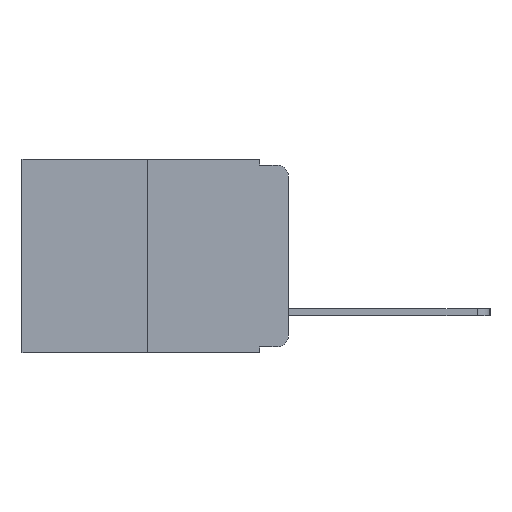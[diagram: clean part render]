
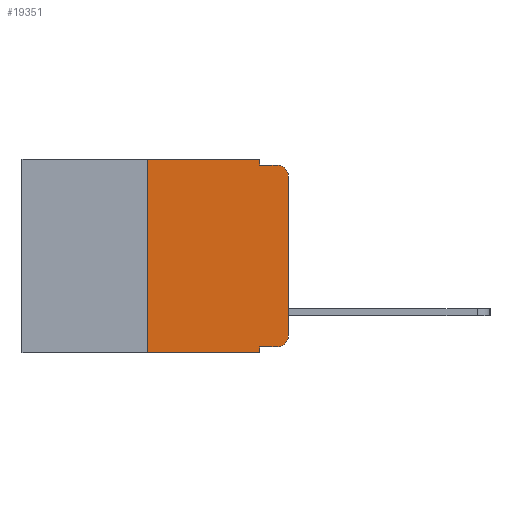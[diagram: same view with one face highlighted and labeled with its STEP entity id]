
A CAD part, left-side view. The second image highlights one B-rep face of the part: STEP entity #19351.
In plain terms, the highlighted planar face has unit normal (-1, 0, 0).
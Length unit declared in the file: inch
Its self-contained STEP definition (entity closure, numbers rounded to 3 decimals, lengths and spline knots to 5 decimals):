
#974 = AXIS2_PLACEMENT_3D ( 'NONE', #1303, #11934, #2923 ) ;
#1007 = LINE ( 'NONE', #12348, #8805 ) ;
#1143 = DIRECTION ( 'NONE',  ( 0., 0., -1. ) ) ;
#1191 = VERTEX_POINT ( 'NONE', #4927 ) ;
#1303 = CARTESIAN_POINT ( 'NONE',  ( 0., 0.02, -0.313 ) ) ;
#1372 = VECTOR ( 'NONE', #17970, 39.37008 ) ;
#1662 = VECTOR ( 'NONE', #10860, 39.37008 ) ;
#1923 = CARTESIAN_POINT ( 'NONE',  ( 0., 0.051, -0.01 ) ) ;
#1928 = CARTESIAN_POINT ( 'NONE',  ( 0., 0.473, -0.343 ) ) ;
#1940 = ORIENTED_EDGE ( 'NONE', *, *, #16941, .F. ) ;
#2173 = LINE ( 'NONE', #13579, #17484 ) ;
#2407 = CIRCLE ( 'NONE', #3943, 0.02 ) ;
#2669 = EDGE_CURVE ( 'NONE', #1191, #8825, #8371, .T. ) ;
#2746 = CARTESIAN_POINT ( 'NONE',  ( 0., 0.02, -0.01 ) ) ;
#2923 = DIRECTION ( 'NONE',  ( 0., 0., -1. ) ) ;
#3154 = CARTESIAN_POINT ( 'NONE',  ( 0., 0.02, -0.03 ) ) ;
#3457 = CARTESIAN_POINT ( 'NONE',  ( 0., 0.051, -0.01 ) ) ;
#3496 = DIRECTION ( 'NONE',  ( 0., -1., 0. ) ) ;
#3943 = AXIS2_PLACEMENT_3D ( 'NONE', #3154, #13618, #4641 ) ;
#4084 = CARTESIAN_POINT ( 'NONE',  ( 0., 0.051, -0.343 ) ) ;
#4249 = VERTEX_POINT ( 'NONE', #13857 ) ;
#4500 = VERTEX_POINT ( 'NONE', #8715 ) ;
#4641 = DIRECTION ( 'NONE',  ( 0., 0., -1. ) ) ;
#4664 = EDGE_CURVE ( 'NONE', #4500, #9839, #13528, .T. ) ;
#4927 = CARTESIAN_POINT ( 'NONE',  ( 0., 0.051, 0. ) ) ;
#6240 = LINE ( 'NONE', #15152, #1662 ) ;
#6700 = VECTOR ( 'NONE', #3496, 39.37008 ) ;
#6738 = EDGE_CURVE ( 'NONE', #19308, #11901, #6240, .T. ) ;
#6889 = ORIENTED_EDGE ( 'NONE', *, *, #17904, .T. ) ;
#7577 = FACE_OUTER_BOUND ( 'NONE', #19037, .T. ) ;
#7788 = CARTESIAN_POINT ( 'NONE',  ( 0., 0., -0.03 ) ) ;
#7885 = VECTOR ( 'NONE', #15950, 39.37008 ) ;
#7889 = CARTESIAN_POINT ( 'NONE',  ( 0., 0.02, -0.333 ) ) ;
#8277 = ORIENTED_EDGE ( 'NONE', *, *, #11507, .T. ) ;
#8371 = LINE ( 'NONE', #15998, #7885 ) ;
#8715 = CARTESIAN_POINT ( 'NONE',  ( 0., 0.25, -0.343 ) ) ;
#8805 = VECTOR ( 'NONE', #13793, 39.37008 ) ;
#8825 = VERTEX_POINT ( 'NONE', #3457 ) ;
#8894 = PLANE ( 'NONE',  #17504 ) ;
#9037 = CARTESIAN_POINT ( 'NONE',  ( 0., 0.25, 0. ) ) ;
#9637 = ORIENTED_EDGE ( 'NONE', *, *, #6738, .F. ) ;
#9698 = VECTOR ( 'NONE', #14856, 39.37008 ) ;
#9839 = VERTEX_POINT ( 'NONE', #16388 ) ;
#10357 = DIRECTION ( 'NONE',  ( 1., 0., 0. ) ) ;
#10398 = CIRCLE ( 'NONE', #974, 0.02 ) ;
#10441 = ORIENTED_EDGE ( 'NONE', *, *, #4664, .F. ) ;
#10860 = DIRECTION ( 'NONE',  ( 0., 0., -1. ) ) ;
#10954 = ORIENTED_EDGE ( 'NONE', *, *, #18392, .F. ) ;
#11170 = LINE ( 'NONE', #1928, #6700 ) ;
#11489 = ORIENTED_EDGE ( 'NONE', *, *, #12147, .T. ) ;
#11507 = EDGE_CURVE ( 'NONE', #4249, #13385, #2173, .T. ) ;
#11901 = VERTEX_POINT ( 'NONE', #4084 ) ;
#11934 = DIRECTION ( 'NONE',  ( -1., 0., 0. ) ) ;
#12008 = ORIENTED_EDGE ( 'NONE', *, *, #13489, .T. ) ;
#12112 = EDGE_CURVE ( 'NONE', #13385, #13826, #2407, .T. ) ;
#12147 = EDGE_CURVE ( 'NONE', #19308, #12839, #13430, .T. ) ;
#12348 = CARTESIAN_POINT ( 'NONE',  ( 0., 0.473, 0. ) ) ;
#12839 = VERTEX_POINT ( 'NONE', #7889 ) ;
#13150 = CARTESIAN_POINT ( 'NONE',  ( 0., 0.051, -0.333 ) ) ;
#13385 = VERTEX_POINT ( 'NONE', #7788 ) ;
#13430 = LINE ( 'NONE', #16572, #1372 ) ;
#13489 = EDGE_CURVE ( 'NONE', #4500, #11901, #11170, .T. ) ;
#13528 = LINE ( 'NONE', #9037, #9698 ) ;
#13579 = CARTESIAN_POINT ( 'NONE',  ( 0., 0., 0. ) ) ;
#13595 = VECTOR ( 'NONE', #13941, 39.37008 ) ;
#13618 = DIRECTION ( 'NONE',  ( -1., 0., 0. ) ) ;
#13793 = DIRECTION ( 'NONE',  ( 0., -1., 0. ) ) ;
#13826 = VERTEX_POINT ( 'NONE', #2746 ) ;
#13857 = CARTESIAN_POINT ( 'NONE',  ( 0., 0., -0.313 ) ) ;
#13941 = DIRECTION ( 'NONE',  ( 0., -1., 0. ) ) ;
#14856 = DIRECTION ( 'NONE',  ( 0., 0., 1. ) ) ;
#15026 = DIRECTION ( 'NONE',  ( 0., 0., 1. ) ) ;
#15152 = CARTESIAN_POINT ( 'NONE',  ( 0., 0.051, 0. ) ) ;
#15879 = ORIENTED_EDGE ( 'NONE', *, *, #2669, .F. ) ;
#15950 = DIRECTION ( 'NONE',  ( 0., 0., -1. ) ) ;
#15998 = CARTESIAN_POINT ( 'NONE',  ( 0., 0.051, 0. ) ) ;
#16388 = CARTESIAN_POINT ( 'NONE',  ( 0., 0.25, 0. ) ) ;
#16572 = CARTESIAN_POINT ( 'NONE',  ( 0., 0.051, -0.333 ) ) ;
#16762 = ORIENTED_EDGE ( 'NONE', *, *, #12112, .T. ) ;
#16941 = EDGE_CURVE ( 'NONE', #8825, #13826, #16967, .T. ) ;
#16967 = LINE ( 'NONE', #1923, #13595 ) ;
#17484 = VECTOR ( 'NONE', #15026, 39.37008 ) ;
#17504 = AXIS2_PLACEMENT_3D ( 'NONE', #18925, #10357, #1143 ) ;
#17904 = EDGE_CURVE ( 'NONE', #12839, #4249, #10398, .T. ) ;
#17970 = DIRECTION ( 'NONE',  ( 0., -1., 0. ) ) ;
#18392 = EDGE_CURVE ( 'NONE', #9839, #1191, #1007, .T. ) ;
#18925 = CARTESIAN_POINT ( 'NONE',  ( 0., 0.473, 0. ) ) ;
#19037 = EDGE_LOOP ( 'NONE', ( #8277, #16762, #1940, #15879, #10954, #10441, #12008, #9637, #11489, #6889 ) ) ;
#19308 = VERTEX_POINT ( 'NONE', #13150 ) ;
#19351 = ADVANCED_FACE ( 'NONE', ( #7577 ), #8894, .F. ) ;
